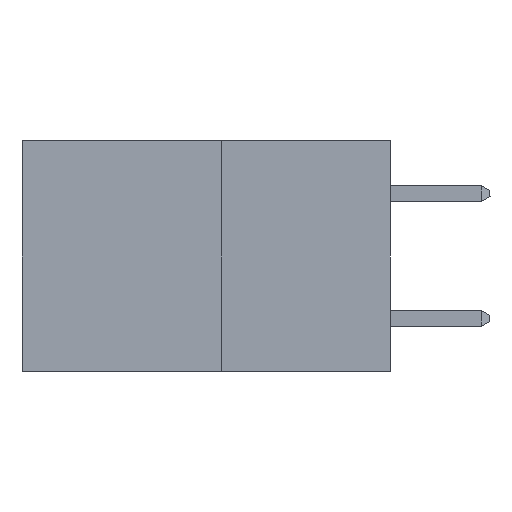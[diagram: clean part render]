
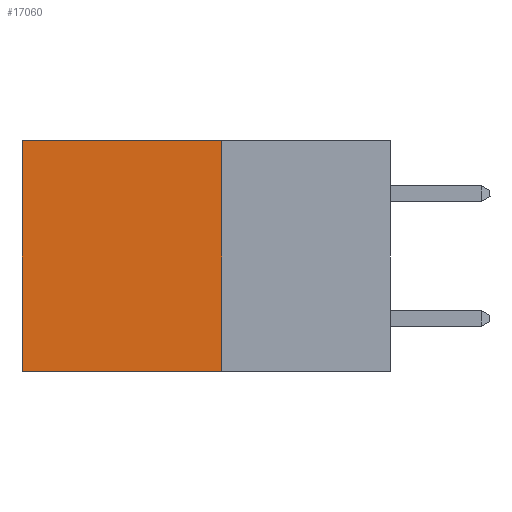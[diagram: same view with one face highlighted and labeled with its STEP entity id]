
A CAD part, left-side view. The second image highlights one B-rep face of the part: STEP entity #17060.
In plain terms, the highlighted planar face has unit normal (-1, 0, 0).
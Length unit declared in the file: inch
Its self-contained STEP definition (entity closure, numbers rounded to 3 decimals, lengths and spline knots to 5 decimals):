
#1586 = VERTEX_POINT ( 'NONE', #12343 ) ;
#1659 = EDGE_CURVE ( 'NONE', #1586, #25094, #15180, .T. ) ;
#3354 = CARTESIAN_POINT ( 'NONE',  ( 0.277, 0.27, -0.37 ) ) ;
#3939 = EDGE_LOOP ( 'NONE', ( #7460, #20490, #9357, #16903 ) ) ;
#3993 = VERTEX_POINT ( 'NONE', #27622 ) ;
#6106 = PLANE ( 'NONE',  #28905 ) ;
#7460 = ORIENTED_EDGE ( 'NONE', *, *, #1659, .T. ) ;
#8024 = VECTOR ( 'NONE', #15190, 39.37008 ) ;
#8776 = DIRECTION ( 'NONE',  ( 0., 0., -1. ) ) ;
#9020 = DIRECTION ( 'NONE',  ( 0., 0., -1. ) ) ;
#9357 = ORIENTED_EDGE ( 'NONE', *, *, #34384, .F. ) ;
#10237 = VECTOR ( 'NONE', #16933, 39.37008 ) ;
#12343 = CARTESIAN_POINT ( 'NONE',  ( 0.277, 0.59, 0. ) ) ;
#15180 = LINE ( 'NONE', #33443, #20771 ) ;
#15190 = DIRECTION ( 'NONE',  ( 0., 0., -1. ) ) ;
#16484 = FACE_OUTER_BOUND ( 'NONE', #3939, .T. ) ;
#16492 = DIRECTION ( 'NONE',  ( 1., 0., 0. ) ) ;
#16903 = ORIENTED_EDGE ( 'NONE', *, *, #24533, .T. ) ;
#16933 = DIRECTION ( 'NONE',  ( 0., 1., 0. ) ) ;
#17060 = ADVANCED_FACE ( 'NONE', ( #16484 ), #6106, .F. ) ;
#18621 = CARTESIAN_POINT ( 'NONE',  ( 0.277, 0.27, 0. ) ) ;
#20490 = ORIENTED_EDGE ( 'NONE', *, *, #32763, .F. ) ;
#20771 = VECTOR ( 'NONE', #9020, 39.37008 ) ;
#22463 = CARTESIAN_POINT ( 'NONE',  ( 0.277, 0.27, 0. ) ) ;
#24496 = CARTESIAN_POINT ( 'NONE',  ( 0.277, 0.59, -0.37 ) ) ;
#24533 = EDGE_CURVE ( 'NONE', #29196, #1586, #33298, .T. ) ;
#24974 = CARTESIAN_POINT ( 'NONE',  ( 0.277, 0.27, -0.37 ) ) ;
#25094 = VERTEX_POINT ( 'NONE', #24496 ) ;
#26234 = VECTOR ( 'NONE', #30357, 39.37008 ) ;
#27622 = CARTESIAN_POINT ( 'NONE',  ( 0.277, 0.27, -0.37 ) ) ;
#28599 = LINE ( 'NONE', #31306, #8024 ) ;
#28905 = AXIS2_PLACEMENT_3D ( 'NONE', #3354, #16492, #8776 ) ;
#29196 = VERTEX_POINT ( 'NONE', #18621 ) ;
#30357 = DIRECTION ( 'NONE',  ( 0., 1., 0. ) ) ;
#31306 = CARTESIAN_POINT ( 'NONE',  ( 0.277, 0.27, -0.37 ) ) ;
#31631 = LINE ( 'NONE', #24974, #10237 ) ;
#32763 = EDGE_CURVE ( 'NONE', #3993, #25094, #31631, .T. ) ;
#33298 = LINE ( 'NONE', #22463, #26234 ) ;
#33443 = CARTESIAN_POINT ( 'NONE',  ( 0.277, 0.59, -0.37 ) ) ;
#34384 = EDGE_CURVE ( 'NONE', #29196, #3993, #28599, .T. ) ;
